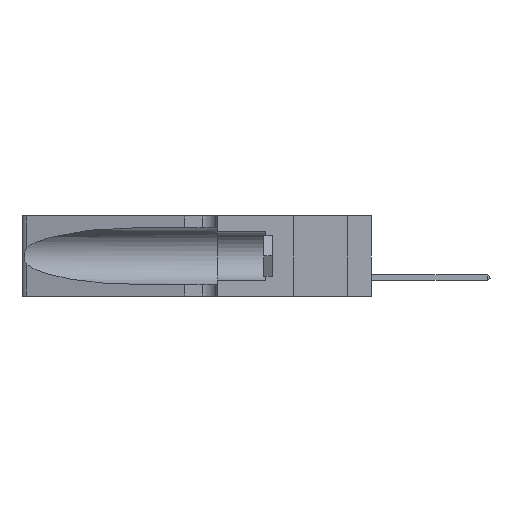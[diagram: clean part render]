
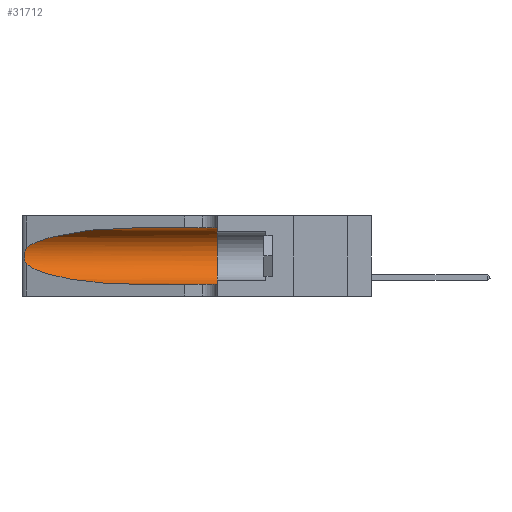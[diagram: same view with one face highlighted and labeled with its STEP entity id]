
A CAD part, left-side view. The second image highlights one B-rep face of the part: STEP entity #31712.
In plain terms, the highlighted cylindrical face has radius 3.308 mm (diameter 6.617 mm), a partial arc.
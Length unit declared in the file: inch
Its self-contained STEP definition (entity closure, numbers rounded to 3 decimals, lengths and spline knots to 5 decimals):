
#1488 = CARTESIAN_POINT ( 'NONE',  ( 0.25487, 1.22718, 0.22369 ) ) ;
#2786 = EDGE_CURVE ( 'NONE', #38421, #22516, #34395, .T. ) ;
#3891 = CARTESIAN_POINT ( 'NONE',  ( 0.1305, 0.35, 0.185 ) ) ;
#4229 = CARTESIAN_POINT ( 'NONE',  ( 0.26075, 1.23896, 0.178 ) ) ;
#4426 = VERTEX_POINT ( 'NONE', #25703 ) ;
#6262 = EDGE_CURVE ( 'NONE', #4426, #38421, #24705, .T. ) ;
#6583 = CARTESIAN_POINT ( 'NONE',  ( 0.25487, 1.22718, 0.14631 ) ) ;
#7799 =( BOUNDED_CURVE ( )  B_SPLINE_CURVE ( 3, ( #39177, #38740, #18528, #25728 ),
 .UNSPECIFIED., .F., .F. ) 
 B_SPLINE_CURVE_WITH_KNOTS ( ( 4, 4 ),
 ( 3.44316, 4.71239 ),
 .UNSPECIFIED. ) 
 CURVE ( )  GEOMETRIC_REPRESENTATION_ITEM ( )  RATIONAL_B_SPLINE_CURVE ( ( 1., 0.87, 0.87, 1. ) ) 
 REPRESENTATION_ITEM ( '' )  );
#7937 = CARTESIAN_POINT ( 'NONE',  ( 0.26075, 1.23896, 0.19203 ) ) ;
#8077 = VERTEX_POINT ( 'NONE', #12826 ) ;
#8688 = ORIENTED_EDGE ( 'NONE', *, *, #9336, .T. ) ;
#9336 = EDGE_CURVE ( 'NONE', #22516, #14817, #7799, .T. ) ;
#11309 = CARTESIAN_POINT ( 'NONE',  ( 0.25789, 1.23486, 0.15765 ) ) ;
#12151 = CARTESIAN_POINT ( 'NONE',  ( 0.2373, 1.15595, 0.28018 ) ) ;
#12404 = DIRECTION ( 'NONE',  ( 0., -1., 0. ) ) ;
#12563 = CARTESIAN_POINT ( 'NONE',  ( 0.1305, 1.61858, 0.31525 ) ) ;
#12826 = CARTESIAN_POINT ( 'NONE',  ( 0.1305, 0.35, 0.31525 ) ) ;
#12867 = FACE_OUTER_BOUND ( 'NONE', #39624, .T. ) ;
#13038 = AXIS2_PLACEMENT_3D ( 'NONE', #42473, #24448, #24735 ) ;
#13324 = VERTEX_POINT ( 'NONE', #22081 ) ;
#14531 = CARTESIAN_POINT ( 'NONE',  ( 0.1305, 1.61858, 0.05475 ) ) ;
#14817 = VERTEX_POINT ( 'NONE', #24998 ) ;
#14880 = CARTESIAN_POINT ( 'NONE',  ( 0.25555, 1.22993, 0.14849 ) ) ;
#15492 = CARTESIAN_POINT ( 'NONE',  ( 0.25487, 1.22718, 0.22369 ) ) ;
#15507 = VECTOR ( 'NONE', #12404, 39.37008 ) ;
#15805 = CIRCLE ( 'NONE', #33171, 0.13025 ) ;
#18528 = CARTESIAN_POINT ( 'NONE',  ( 0.18966, 0.96281, 0.05475 ) ) ;
#19016 = CARTESIAN_POINT ( 'NONE',  ( 0.25787, 1.23484, 0.2124 ) ) ;
#20565 = CYLINDRICAL_SURFACE ( 'NONE', #13038, 0.13025 ) ;
#22061 = CARTESIAN_POINT ( 'NONE',  ( 0.26017, 1.23833, 0.17102 ) ) ;
#22081 = CARTESIAN_POINT ( 'NONE',  ( 0.1305, 0.35, 0.05475 ) ) ;
#22516 = VERTEX_POINT ( 'NONE', #6583 ) ;
#22913 = CARTESIAN_POINT ( 'NONE',  ( 0.18966, 0.96281, 0.31525 ) ) ;
#23888 = LINE ( 'NONE', #14531, #24943 ) ;
#24448 = DIRECTION ( 'NONE',  ( 0., -1., 0. ) ) ;
#24705 =( BOUNDED_CURVE ( )  B_SPLINE_CURVE ( 3, ( #44047, #22913, #12151, #1488 ),
 .UNSPECIFIED., .F., .T. ) 
 B_SPLINE_CURVE_WITH_KNOTS ( ( 4, 4 ),
 ( 1.5708, 2.84003 ),
 .UNSPECIFIED. ) 
 CURVE ( )  GEOMETRIC_REPRESENTATION_ITEM ( )  RATIONAL_B_SPLINE_CURVE ( ( 1., 0.87, 0.87, 1. ) ) 
 REPRESENTATION_ITEM ( '' )  );
#24735 = DIRECTION ( 'NONE',  ( 0., 0., -1. ) ) ;
#24815 = LINE ( 'NONE', #12563, #15507 ) ;
#24943 = VECTOR ( 'NONE', #39157, 39.37008 ) ;
#24998 = CARTESIAN_POINT ( 'NONE',  ( 0.1305, 0.72297, 0.05475 ) ) ;
#25287 = CARTESIAN_POINT ( 'NONE',  ( 0.25854, 1.2359, 0.20912 ) ) ;
#25703 = CARTESIAN_POINT ( 'NONE',  ( 0.1305, 0.72297, 0.31525 ) ) ;
#25728 = CARTESIAN_POINT ( 'NONE',  ( 0.1305, 0.72297, 0.05475 ) ) ;
#26633 = ORIENTED_EDGE ( 'NONE', *, *, #38888, .T. ) ;
#28837 = CARTESIAN_POINT ( 'NONE',  ( 0.25856, 1.23593, 0.16098 ) ) ;
#31712 = ADVANCED_FACE ( 'NONE', ( #12867 ), #20565, .F. ) ;
#32395 = CARTESIAN_POINT ( 'NONE',  ( 0.25639, 1.23184, 0.21858 ) ) ;
#32497 = ORIENTED_EDGE ( 'NONE', *, *, #6262, .T. ) ;
#33171 = AXIS2_PLACEMENT_3D ( 'NONE', #3891, #42551, #39024 ) ;
#34395 = B_SPLINE_CURVE_WITH_KNOTS ( 'NONE', 3,
 ( #15492, #40143, #32395, #19016, #25287, #43695, #7937, #4229, #22061, #28837, #11309, #35965, #14880, #43066 ),
 .UNSPECIFIED., .F., .F.,
 ( 4, 2, 2, 2, 2, 2, 4 ),
 ( 0., 0.00027, 0.00053, 0.00107, 0.0016, 0.00187, 0.00214 ),
 .UNSPECIFIED. ) ;
#35225 = EDGE_CURVE ( 'NONE', #8077, #13324, #15805, .T. ) ;
#35965 = CARTESIAN_POINT ( 'NONE',  ( 0.25639, 1.23186, 0.15144 ) ) ;
#37755 = CARTESIAN_POINT ( 'NONE',  ( 0.25487, 1.22718, 0.22369 ) ) ;
#37873 = ORIENTED_EDGE ( 'NONE', *, *, #35225, .F. ) ;
#38115 = ORIENTED_EDGE ( 'NONE', *, *, #2786, .T. ) ;
#38421 = VERTEX_POINT ( 'NONE', #37755 ) ;
#38740 = CARTESIAN_POINT ( 'NONE',  ( 0.2373, 1.15595, 0.08982 ) ) ;
#38888 = EDGE_CURVE ( 'NONE', #14817, #13324, #23888, .T. ) ;
#39024 = DIRECTION ( 'NONE',  ( 0., 0., 1. ) ) ;
#39157 = DIRECTION ( 'NONE',  ( 0., -1., 0. ) ) ;
#39177 = CARTESIAN_POINT ( 'NONE',  ( 0.25487, 1.22718, 0.14631 ) ) ;
#39624 = EDGE_LOOP ( 'NONE', ( #32497, #38115, #8688, #26633, #37873, #43099 ) ) ;
#40143 = CARTESIAN_POINT ( 'NONE',  ( 0.25555, 1.22994, 0.2215 ) ) ;
#40179 = EDGE_CURVE ( 'NONE', #4426, #8077, #24815, .T. ) ;
#42473 = CARTESIAN_POINT ( 'NONE',  ( 0.1305, 1.61858, 0.185 ) ) ;
#42551 = DIRECTION ( 'NONE',  ( 0., 1., 0. ) ) ;
#43066 = CARTESIAN_POINT ( 'NONE',  ( 0.25487, 1.22718, 0.14631 ) ) ;
#43099 = ORIENTED_EDGE ( 'NONE', *, *, #40179, .F. ) ;
#43695 = CARTESIAN_POINT ( 'NONE',  ( 0.26018, 1.23835, 0.19895 ) ) ;
#44047 = CARTESIAN_POINT ( 'NONE',  ( 0.1305, 0.72297, 0.31525 ) ) ;
